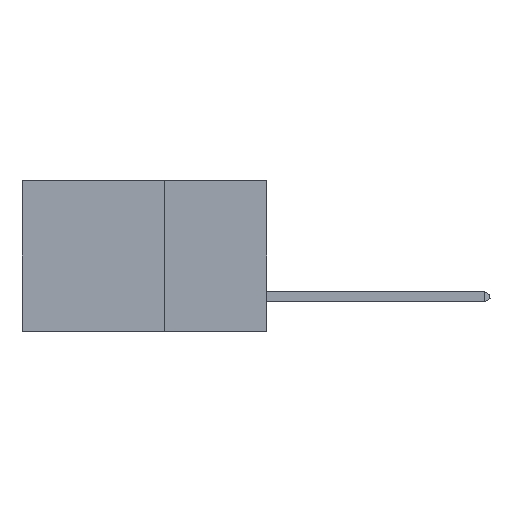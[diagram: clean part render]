
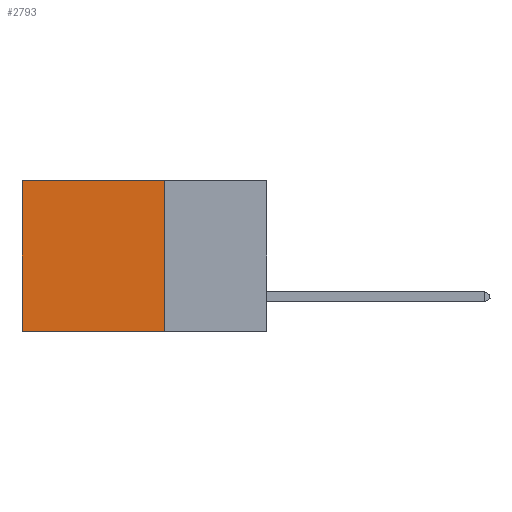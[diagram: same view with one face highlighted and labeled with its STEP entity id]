
A CAD part, left-side view. The second image highlights one B-rep face of the part: STEP entity #2793.
In plain terms, the highlighted planar face has unit normal (-1, 0, 0).
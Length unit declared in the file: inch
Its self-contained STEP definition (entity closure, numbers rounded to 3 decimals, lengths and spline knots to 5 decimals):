
#752 = DIRECTION ( 'NONE',  ( 0., 1., 0. ) ) ;
#1559 = CARTESIAN_POINT ( 'NONE',  ( 0.2875, 0.25, -0.37 ) ) ;
#2793 = ADVANCED_FACE ( 'NONE', ( #29608 ), #23647, .F. ) ;
#5017 = VERTEX_POINT ( 'NONE', #34094 ) ;
#8887 = ORIENTED_EDGE ( 'NONE', *, *, #36315, .F. ) ;
#11035 = VECTOR ( 'NONE', #36877, 39.37008 ) ;
#13160 = ORIENTED_EDGE ( 'NONE', *, *, #27365, .T. ) ;
#14139 = VECTOR ( 'NONE', #752, 39.37008 ) ;
#15074 = LINE ( 'NONE', #25050, #14139 ) ;
#15092 = ORIENTED_EDGE ( 'NONE', *, *, #15342, .T. ) ;
#15342 = EDGE_CURVE ( 'NONE', #21651, #19031, #37814, .T. ) ;
#17986 = VECTOR ( 'NONE', #29575, 39.37008 ) ;
#19031 = VERTEX_POINT ( 'NONE', #19475 ) ;
#19068 = CARTESIAN_POINT ( 'NONE',  ( 0.2875, 0.25, 0. ) ) ;
#19475 = CARTESIAN_POINT ( 'NONE',  ( 0.2875, 0.6, -0.37 ) ) ;
#19960 = EDGE_CURVE ( 'NONE', #5017, #25918, #26145, .T. ) ;
#20186 = CARTESIAN_POINT ( 'NONE',  ( 0.2875, 0.6, 0. ) ) ;
#21194 = EDGE_LOOP ( 'NONE', ( #15092, #8887, #32874, #13160 ) ) ;
#21393 = DIRECTION ( 'NONE',  ( 0., 0., -1. ) ) ;
#21651 = VERTEX_POINT ( 'NONE', #20186 ) ;
#21760 = AXIS2_PLACEMENT_3D ( 'NONE', #22800, #22547, #22493 ) ;
#22493 = DIRECTION ( 'NONE',  ( 0., 0., -1. ) ) ;
#22547 = DIRECTION ( 'NONE',  ( 1., 0., 0. ) ) ;
#22800 = CARTESIAN_POINT ( 'NONE',  ( 0.2875, 0.25, 0. ) ) ;
#23618 = CARTESIAN_POINT ( 'NONE',  ( 0.2875, 0.25, 0. ) ) ;
#23647 = PLANE ( 'NONE',  #21760 ) ;
#25050 = CARTESIAN_POINT ( 'NONE',  ( 0.2875, 0.25, -0.37 ) ) ;
#25918 = VERTEX_POINT ( 'NONE', #1559 ) ;
#26145 = LINE ( 'NONE', #19068, #11035 ) ;
#27365 = EDGE_CURVE ( 'NONE', #5017, #21651, #32904, .T. ) ;
#29575 = DIRECTION ( 'NONE',  ( 0., 1., 0. ) ) ;
#29608 = FACE_OUTER_BOUND ( 'NONE', #21194, .T. ) ;
#30849 = VECTOR ( 'NONE', #21393, 39.37008 ) ;
#32874 = ORIENTED_EDGE ( 'NONE', *, *, #19960, .F. ) ;
#32904 = LINE ( 'NONE', #23618, #17986 ) ;
#34094 = CARTESIAN_POINT ( 'NONE',  ( 0.2875, 0.25, 0. ) ) ;
#36194 = CARTESIAN_POINT ( 'NONE',  ( 0.2875, 0.6, 0. ) ) ;
#36315 = EDGE_CURVE ( 'NONE', #25918, #19031, #15074, .T. ) ;
#36877 = DIRECTION ( 'NONE',  ( 0., 0., -1. ) ) ;
#37814 = LINE ( 'NONE', #36194, #30849 ) ;
